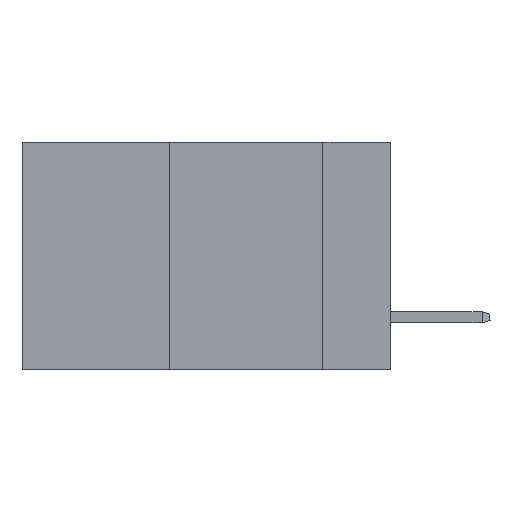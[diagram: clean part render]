
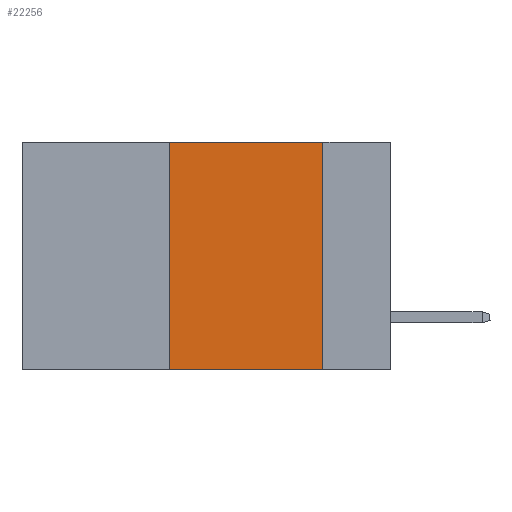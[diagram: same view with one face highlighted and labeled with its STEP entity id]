
A CAD part, left-side view. The second image highlights one B-rep face of the part: STEP entity #22256.
In plain terms, the highlighted planar face has unit normal (-1, 0, 0).
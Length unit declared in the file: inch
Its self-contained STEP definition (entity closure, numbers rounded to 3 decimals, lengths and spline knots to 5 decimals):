
#752 = LINE ( 'NONE', #27521, #46375 ) ;
#7114 = EDGE_CURVE ( 'NONE', #17554, #40891, #48147, .T. ) ;
#7707 = ORIENTED_EDGE ( 'NONE', *, *, #7114, .F. ) ;
#7880 = CARTESIAN_POINT ( 'NONE',  ( 0., 0.36, -0.37 ) ) ;
#8216 = DIRECTION ( 'NONE',  ( 0., -1., 0. ) ) ;
#10497 = EDGE_LOOP ( 'NONE', ( #33015, #7707, #20717, #14187 ) ) ;
#11941 = PLANE ( 'NONE',  #47730 ) ;
#11970 = DIRECTION ( 'NONE',  ( 0., 0., -1. ) ) ;
#14187 = ORIENTED_EDGE ( 'NONE', *, *, #18431, .T. ) ;
#15701 = VECTOR ( 'NONE', #21524, 39.37008 ) ;
#15858 = DIRECTION ( 'NONE',  ( 1., 0., 0. ) ) ;
#16219 = CARTESIAN_POINT ( 'NONE',  ( 0., 0.11, 0. ) ) ;
#16743 = CARTESIAN_POINT ( 'NONE',  ( 0., 0.6, 0. ) ) ;
#17554 = VERTEX_POINT ( 'NONE', #30873 ) ;
#18431 = EDGE_CURVE ( 'NONE', #34246, #42695, #752, .T. ) ;
#19414 = VECTOR ( 'NONE', #39333, 39.37008 ) ;
#19594 = EDGE_CURVE ( 'NONE', #34246, #17554, #44448, .T. ) ;
#20717 = ORIENTED_EDGE ( 'NONE', *, *, #19594, .F. ) ;
#21524 = DIRECTION ( 'NONE',  ( 0., 0., 1. ) ) ;
#22135 = LINE ( 'NONE', #16219, #43227 ) ;
#22256 = ADVANCED_FACE ( 'NONE', ( #28934 ), #11941, .F. ) ;
#23047 = CARTESIAN_POINT ( 'NONE',  ( 0., 0.6, 0. ) ) ;
#26798 = CARTESIAN_POINT ( 'NONE',  ( 0., 0.11, -0.37 ) ) ;
#26883 = CARTESIAN_POINT ( 'NONE',  ( 0., 0.36, 0. ) ) ;
#27521 = CARTESIAN_POINT ( 'NONE',  ( 0., 0.6, -0.37 ) ) ;
#28934 = FACE_OUTER_BOUND ( 'NONE', #10497, .T. ) ;
#30321 = EDGE_CURVE ( 'NONE', #40891, #42695, #22135, .T. ) ;
#30873 = CARTESIAN_POINT ( 'NONE',  ( 0., 0.36, 0. ) ) ;
#33015 = ORIENTED_EDGE ( 'NONE', *, *, #30321, .F. ) ;
#34246 = VERTEX_POINT ( 'NONE', #7880 ) ;
#35522 = DIRECTION ( 'NONE',  ( 0., 0., -1. ) ) ;
#39333 = DIRECTION ( 'NONE',  ( 0., -1., 0. ) ) ;
#40891 = VERTEX_POINT ( 'NONE', #41596 ) ;
#41596 = CARTESIAN_POINT ( 'NONE',  ( 0., 0.11, 0. ) ) ;
#42695 = VERTEX_POINT ( 'NONE', #26798 ) ;
#43227 = VECTOR ( 'NONE', #11970, 39.37008 ) ;
#44448 = LINE ( 'NONE', #26883, #15701 ) ;
#46375 = VECTOR ( 'NONE', #8216, 39.37008 ) ;
#47730 = AXIS2_PLACEMENT_3D ( 'NONE', #23047, #15858, #35522 ) ;
#48147 = LINE ( 'NONE', #16743, #19414 ) ;
